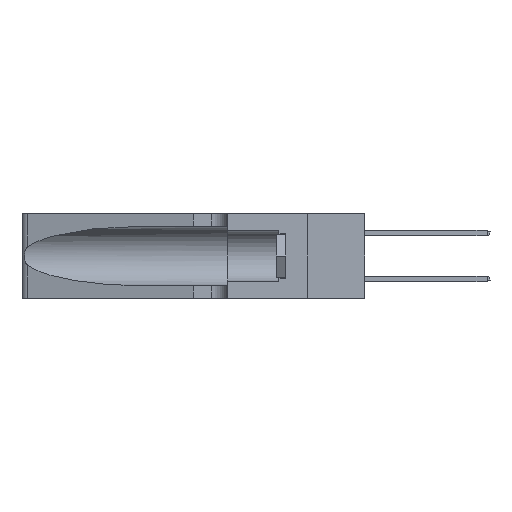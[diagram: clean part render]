
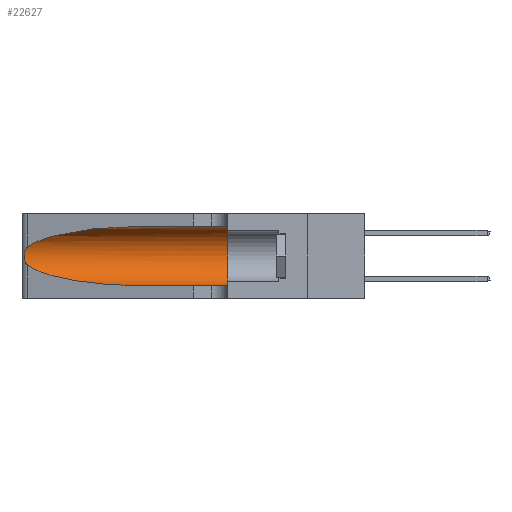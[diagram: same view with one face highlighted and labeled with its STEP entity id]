
A CAD part, left-side view. The second image highlights one B-rep face of the part: STEP entity #22627.
In plain terms, the highlighted cylindrical face has radius 3.308 mm (diameter 6.617 mm), a partial arc.
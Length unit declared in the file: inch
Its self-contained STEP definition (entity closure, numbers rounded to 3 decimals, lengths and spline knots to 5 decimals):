
#269 = VERTEX_POINT ( 'NONE', #17822 ) ;
#1120 = LINE ( 'NONE', #11207, #26281 ) ;
#1553 = CARTESIAN_POINT ( 'NONE',  ( 0.25787, 1.23484, 0.2124 ) ) ;
#2115 = VECTOR ( 'NONE', #21627, 39.37008 ) ;
#2304 =( BOUNDED_CURVE ( )  B_SPLINE_CURVE ( 3, ( #29031, #14952, #5631, #22060 ),
 .UNSPECIFIED., .F., .F. ) 
 B_SPLINE_CURVE_WITH_KNOTS ( ( 4, 4 ),
 ( 3.44316, 4.71239 ),
 .UNSPECIFIED. ) 
 CURVE ( )  GEOMETRIC_REPRESENTATION_ITEM ( )  RATIONAL_B_SPLINE_CURVE ( ( 1., 0.87, 0.87, 1. ) ) 
 REPRESENTATION_ITEM ( '' )  );
#3520 = VERTEX_POINT ( 'NONE', #17327 ) ;
#4005 = CARTESIAN_POINT ( 'NONE',  ( 0.26018, 1.23835, 0.19895 ) ) ;
#5607 = B_SPLINE_CURVE_WITH_KNOTS ( 'NONE', 3,
 ( #27467, #29811, #15742, #1553, #18124, #4005, #20462, #6409, #22841, #8753, #25197, #11126, #27563, #13490 ),
 .UNSPECIFIED., .F., .F.,
 ( 4, 2, 2, 2, 2, 2, 4 ),
 ( 0., 0.00027, 0.00053, 0.00107, 0.0016, 0.00187, 0.00214 ),
 .UNSPECIFIED. ) ;
#5631 = CARTESIAN_POINT ( 'NONE',  ( 0.18966, 0.96281, 0.05475 ) ) ;
#5849 = FACE_OUTER_BOUND ( 'NONE', #18268, .T. ) ;
#6409 = CARTESIAN_POINT ( 'NONE',  ( 0.26075, 1.23896, 0.178 ) ) ;
#6894 = CARTESIAN_POINT ( 'NONE',  ( 0.1305, 0.35, 0.185 ) ) ;
#7648 = ORIENTED_EDGE ( 'NONE', *, *, #12782, .T. ) ;
#7862 =( BOUNDED_CURVE ( )  B_SPLINE_CURVE ( 3, ( #25684, #16230, #30376, #16321 ),
 .UNSPECIFIED., .F., .T. ) 
 B_SPLINE_CURVE_WITH_KNOTS ( ( 4, 4 ),
 ( 1.5708, 2.84003 ),
 .UNSPECIFIED. ) 
 CURVE ( )  GEOMETRIC_REPRESENTATION_ITEM ( )  RATIONAL_B_SPLINE_CURVE ( ( 1., 0.87, 0.87, 1. ) ) 
 REPRESENTATION_ITEM ( '' )  );
#8637 = ORIENTED_EDGE ( 'NONE', *, *, #30353, .F. ) ;
#8753 = CARTESIAN_POINT ( 'NONE',  ( 0.25856, 1.23593, 0.16098 ) ) ;
#8945 = VERTEX_POINT ( 'NONE', #20335 ) ;
#9269 = DIRECTION ( 'NONE',  ( 0., 0., 1. ) ) ;
#10951 = AXIS2_PLACEMENT_3D ( 'NONE', #6894, #23342, #9269 ) ;
#11126 = CARTESIAN_POINT ( 'NONE',  ( 0.25639, 1.23186, 0.15144 ) ) ;
#11207 = CARTESIAN_POINT ( 'NONE',  ( 0.1305, 1.61858, 0.05475 ) ) ;
#12782 = EDGE_CURVE ( 'NONE', #28501, #8945, #7862, .T. ) ;
#12874 = VERTEX_POINT ( 'NONE', #23721 ) ;
#12991 = CARTESIAN_POINT ( 'NONE',  ( 0.1305, 1.61858, 0.185 ) ) ;
#13060 = EDGE_CURVE ( 'NONE', #3520, #269, #2304, .T. ) ;
#13092 = DIRECTION ( 'NONE',  ( 0., 0., -1. ) ) ;
#13490 = CARTESIAN_POINT ( 'NONE',  ( 0.25487, 1.22718, 0.14631 ) ) ;
#13560 = DIRECTION ( 'NONE',  ( 0., -1., 0. ) ) ;
#13868 = CIRCLE ( 'NONE', #10951, 0.13025 ) ;
#14952 = CARTESIAN_POINT ( 'NONE',  ( 0.2373, 1.15595, 0.08982 ) ) ;
#15424 = DIRECTION ( 'NONE',  ( 0., -1., 0. ) ) ;
#15742 = CARTESIAN_POINT ( 'NONE',  ( 0.25639, 1.23184, 0.21858 ) ) ;
#16230 = CARTESIAN_POINT ( 'NONE',  ( 0.18966, 0.96281, 0.31525 ) ) ;
#16321 = CARTESIAN_POINT ( 'NONE',  ( 0.25487, 1.22718, 0.22369 ) ) ;
#17327 = CARTESIAN_POINT ( 'NONE',  ( 0.25487, 1.22718, 0.14631 ) ) ;
#17822 = CARTESIAN_POINT ( 'NONE',  ( 0.1305, 0.72297, 0.05475 ) ) ;
#18124 = CARTESIAN_POINT ( 'NONE',  ( 0.25854, 1.2359, 0.20912 ) ) ;
#18268 = EDGE_LOOP ( 'NONE', ( #7648, #27212, #22803, #18525, #22642, #8637 ) ) ;
#18400 = VERTEX_POINT ( 'NONE', #24919 ) ;
#18525 = ORIENTED_EDGE ( 'NONE', *, *, #28164, .T. ) ;
#19067 = EDGE_CURVE ( 'NONE', #8945, #3520, #5607, .T. ) ;
#19295 = CARTESIAN_POINT ( 'NONE',  ( 0.1305, 0.72297, 0.31525 ) ) ;
#20335 = CARTESIAN_POINT ( 'NONE',  ( 0.25487, 1.22718, 0.22369 ) ) ;
#20462 = CARTESIAN_POINT ( 'NONE',  ( 0.26075, 1.23896, 0.19203 ) ) ;
#21627 = DIRECTION ( 'NONE',  ( 0., -1., 0. ) ) ;
#22060 = CARTESIAN_POINT ( 'NONE',  ( 0.1305, 0.72297, 0.05475 ) ) ;
#22109 = AXIS2_PLACEMENT_3D ( 'NONE', #12991, #15424, #13092 ) ;
#22627 = ADVANCED_FACE ( 'NONE', ( #5849 ), #23860, .F. ) ;
#22642 = ORIENTED_EDGE ( 'NONE', *, *, #26375, .F. ) ;
#22803 = ORIENTED_EDGE ( 'NONE', *, *, #13060, .T. ) ;
#22841 = CARTESIAN_POINT ( 'NONE',  ( 0.26017, 1.23833, 0.17102 ) ) ;
#23342 = DIRECTION ( 'NONE',  ( 0., 1., 0. ) ) ;
#23721 = CARTESIAN_POINT ( 'NONE',  ( 0.1305, 0.35, 0.31525 ) ) ;
#23860 = CYLINDRICAL_SURFACE ( 'NONE', #22109, 0.13025 ) ;
#24919 = CARTESIAN_POINT ( 'NONE',  ( 0.1305, 0.35, 0.05475 ) ) ;
#25197 = CARTESIAN_POINT ( 'NONE',  ( 0.25789, 1.23486, 0.15765 ) ) ;
#25684 = CARTESIAN_POINT ( 'NONE',  ( 0.1305, 0.72297, 0.31525 ) ) ;
#26281 = VECTOR ( 'NONE', #13560, 39.37008 ) ;
#26287 = CARTESIAN_POINT ( 'NONE',  ( 0.1305, 1.61858, 0.31525 ) ) ;
#26375 = EDGE_CURVE ( 'NONE', #12874, #18400, #13868, .T. ) ;
#27212 = ORIENTED_EDGE ( 'NONE', *, *, #19067, .T. ) ;
#27467 = CARTESIAN_POINT ( 'NONE',  ( 0.25487, 1.22718, 0.22369 ) ) ;
#27563 = CARTESIAN_POINT ( 'NONE',  ( 0.25555, 1.22993, 0.14849 ) ) ;
#27932 = LINE ( 'NONE', #26287, #2115 ) ;
#28164 = EDGE_CURVE ( 'NONE', #269, #18400, #1120, .T. ) ;
#28501 = VERTEX_POINT ( 'NONE', #19295 ) ;
#29031 = CARTESIAN_POINT ( 'NONE',  ( 0.25487, 1.22718, 0.14631 ) ) ;
#29811 = CARTESIAN_POINT ( 'NONE',  ( 0.25555, 1.22994, 0.2215 ) ) ;
#30353 = EDGE_CURVE ( 'NONE', #28501, #12874, #27932, .T. ) ;
#30376 = CARTESIAN_POINT ( 'NONE',  ( 0.2373, 1.15595, 0.28018 ) ) ;
